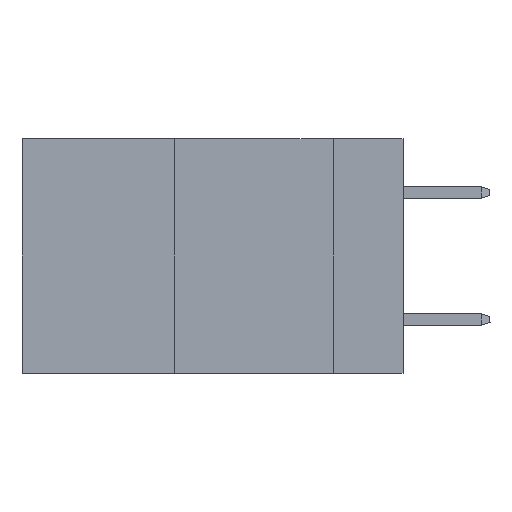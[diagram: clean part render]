
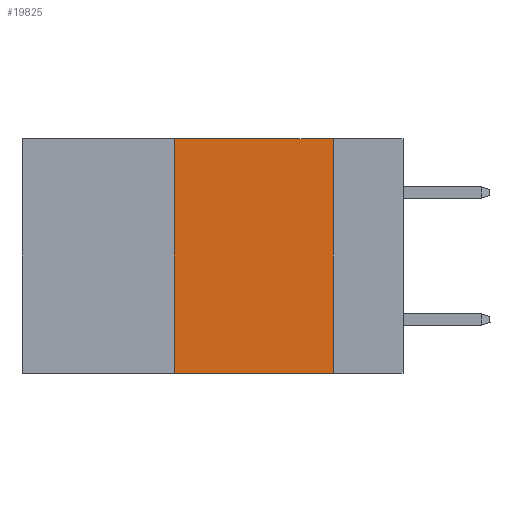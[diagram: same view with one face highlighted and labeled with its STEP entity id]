
A CAD part, left-side view. The second image highlights one B-rep face of the part: STEP entity #19825.
In plain terms, the highlighted planar face has unit normal (-1, 0, 0).
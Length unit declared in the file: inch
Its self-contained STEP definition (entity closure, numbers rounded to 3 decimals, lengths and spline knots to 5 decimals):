
#221 = VERTEX_POINT ( 'NONE', #21257 ) ;
#266 = EDGE_CURVE ( 'NONE', #221, #17859, #1359, .T. ) ;
#1359 = LINE ( 'NONE', #22704, #7749 ) ;
#2559 = DIRECTION ( 'NONE',  ( 0., 0., -1. ) ) ;
#4082 = EDGE_CURVE ( 'NONE', #17859, #5180, #14963, .T. ) ;
#5180 = VERTEX_POINT ( 'NONE', #16113 ) ;
#7339 = CARTESIAN_POINT ( 'NONE',  ( 0., 0.36, -0.37 ) ) ;
#7507 = LINE ( 'NONE', #9638, #15049 ) ;
#7743 = DIRECTION ( 'NONE',  ( 0., 0., 1. ) ) ;
#7749 = VECTOR ( 'NONE', #15818, 39.37008 ) ;
#8647 = ORIENTED_EDGE ( 'NONE', *, *, #266, .F. ) ;
#8906 = LINE ( 'NONE', #13977, #16461 ) ;
#9393 = CARTESIAN_POINT ( 'NONE',  ( 0., 0.11, 0. ) ) ;
#9638 = CARTESIAN_POINT ( 'NONE',  ( 0., 0.36, 0. ) ) ;
#11291 = DIRECTION ( 'NONE',  ( 0., 0., -1. ) ) ;
#11587 = CARTESIAN_POINT ( 'NONE',  ( 0., 0.6, 0. ) ) ;
#13332 = EDGE_CURVE ( 'NONE', #13402, #5180, #8906, .T. ) ;
#13402 = VERTEX_POINT ( 'NONE', #7339 ) ;
#13554 = ORIENTED_EDGE ( 'NONE', *, *, #18750, .F. ) ;
#13977 = CARTESIAN_POINT ( 'NONE',  ( 0., 0.6, -0.37 ) ) ;
#14963 = LINE ( 'NONE', #9393, #21988 ) ;
#15049 = VECTOR ( 'NONE', #7743, 39.37008 ) ;
#15138 = PLANE ( 'NONE',  #15925 ) ;
#15818 = DIRECTION ( 'NONE',  ( 0., -1., 0. ) ) ;
#15925 = AXIS2_PLACEMENT_3D ( 'NONE', #11587, #18834, #2559 ) ;
#16047 = ORIENTED_EDGE ( 'NONE', *, *, #13332, .T. ) ;
#16113 = CARTESIAN_POINT ( 'NONE',  ( 0., 0.11, -0.37 ) ) ;
#16461 = VECTOR ( 'NONE', #17533, 39.37008 ) ;
#17029 = ORIENTED_EDGE ( 'NONE', *, *, #4082, .F. ) ;
#17533 = DIRECTION ( 'NONE',  ( 0., -1., 0. ) ) ;
#17859 = VERTEX_POINT ( 'NONE', #20710 ) ;
#18495 = EDGE_LOOP ( 'NONE', ( #17029, #8647, #13554, #16047 ) ) ;
#18750 = EDGE_CURVE ( 'NONE', #13402, #221, #7507, .T. ) ;
#18834 = DIRECTION ( 'NONE',  ( 1., 0., 0. ) ) ;
#19825 = ADVANCED_FACE ( 'NONE', ( #21130 ), #15138, .F. ) ;
#20710 = CARTESIAN_POINT ( 'NONE',  ( 0., 0.11, 0. ) ) ;
#21130 = FACE_OUTER_BOUND ( 'NONE', #18495, .T. ) ;
#21257 = CARTESIAN_POINT ( 'NONE',  ( 0., 0.36, 0. ) ) ;
#21988 = VECTOR ( 'NONE', #11291, 39.37008 ) ;
#22704 = CARTESIAN_POINT ( 'NONE',  ( 0., 0.6, 0. ) ) ;
